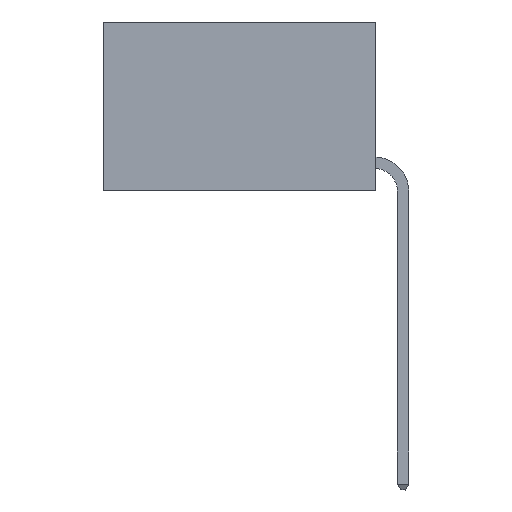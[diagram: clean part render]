
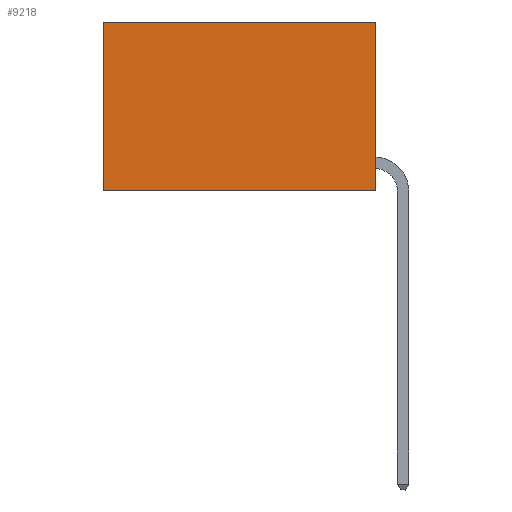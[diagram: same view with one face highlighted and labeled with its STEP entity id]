
A CAD part, left-side view. The second image highlights one B-rep face of the part: STEP entity #9218.
In plain terms, the highlighted planar face has unit normal (-1, 0, 0).
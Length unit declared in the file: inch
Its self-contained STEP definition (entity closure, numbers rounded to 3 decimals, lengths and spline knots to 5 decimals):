
#455 = CARTESIAN_POINT ( 'NONE',  ( 0.2625, 0., 0. ) ) ;
#843 = VERTEX_POINT ( 'NONE', #2199 ) ;
#1808 = LINE ( 'NONE', #9470, #12782 ) ;
#2199 = CARTESIAN_POINT ( 'NONE',  ( 0.2625, 0.6, -0.37 ) ) ;
#2541 = VECTOR ( 'NONE', #16073, 39.37008 ) ;
#4657 = CARTESIAN_POINT ( 'NONE',  ( 0.2625, 0., 0. ) ) ;
#6047 = ORIENTED_EDGE ( 'NONE', *, *, #17116, .T. ) ;
#6233 = VERTEX_POINT ( 'NONE', #27560 ) ;
#6280 = FACE_OUTER_BOUND ( 'NONE', #20027, .T. ) ;
#6403 = ORIENTED_EDGE ( 'NONE', *, *, #8672, .F. ) ;
#6978 = CARTESIAN_POINT ( 'NONE',  ( 0.2625, 0.6, 0. ) ) ;
#8620 = LINE ( 'NONE', #6978, #9302 ) ;
#8672 = EDGE_CURVE ( 'NONE', #24456, #843, #14870, .T. ) ;
#8949 = PLANE ( 'NONE',  #21529 ) ;
#9218 = ADVANCED_FACE ( 'NONE', ( #6280 ), #8949, .F. ) ;
#9262 = EDGE_CURVE ( 'NONE', #6233, #24293, #10016, .T. ) ;
#9302 = VECTOR ( 'NONE', #13489, 39.37008 ) ;
#9470 = CARTESIAN_POINT ( 'NONE',  ( 0.2625, 0., 0. ) ) ;
#10016 = LINE ( 'NONE', #455, #15184 ) ;
#11253 = DIRECTION ( 'NONE',  ( 1., 0., 0. ) ) ;
#11676 = DIRECTION ( 'NONE',  ( 0., 0., -1. ) ) ;
#12782 = VECTOR ( 'NONE', #11676, 39.37008 ) ;
#13489 = DIRECTION ( 'NONE',  ( 0., 0., -1. ) ) ;
#13669 = ORIENTED_EDGE ( 'NONE', *, *, #16545, .F. ) ;
#13875 = CARTESIAN_POINT ( 'NONE',  ( 0.2625, 0., -0.37 ) ) ;
#14261 = CARTESIAN_POINT ( 'NONE',  ( 0.2625, 0., -0.37 ) ) ;
#14870 = LINE ( 'NONE', #13875, #2541 ) ;
#15184 = VECTOR ( 'NONE', #26323, 39.37008 ) ;
#16073 = DIRECTION ( 'NONE',  ( 0., 1., 0. ) ) ;
#16545 = EDGE_CURVE ( 'NONE', #6233, #24456, #1808, .T. ) ;
#17116 = EDGE_CURVE ( 'NONE', #24293, #843, #8620, .T. ) ;
#20027 = EDGE_LOOP ( 'NONE', ( #6047, #6403, #13669, #26895 ) ) ;
#21529 = AXIS2_PLACEMENT_3D ( 'NONE', #4657, #11253, #26150 ) ;
#24293 = VERTEX_POINT ( 'NONE', #26472 ) ;
#24456 = VERTEX_POINT ( 'NONE', #14261 ) ;
#26150 = DIRECTION ( 'NONE',  ( 0., 0., -1. ) ) ;
#26323 = DIRECTION ( 'NONE',  ( 0., 1., 0. ) ) ;
#26472 = CARTESIAN_POINT ( 'NONE',  ( 0.2625, 0.6, 0. ) ) ;
#26895 = ORIENTED_EDGE ( 'NONE', *, *, #9262, .T. ) ;
#27560 = CARTESIAN_POINT ( 'NONE',  ( 0.2625, 0., 0. ) ) ;
